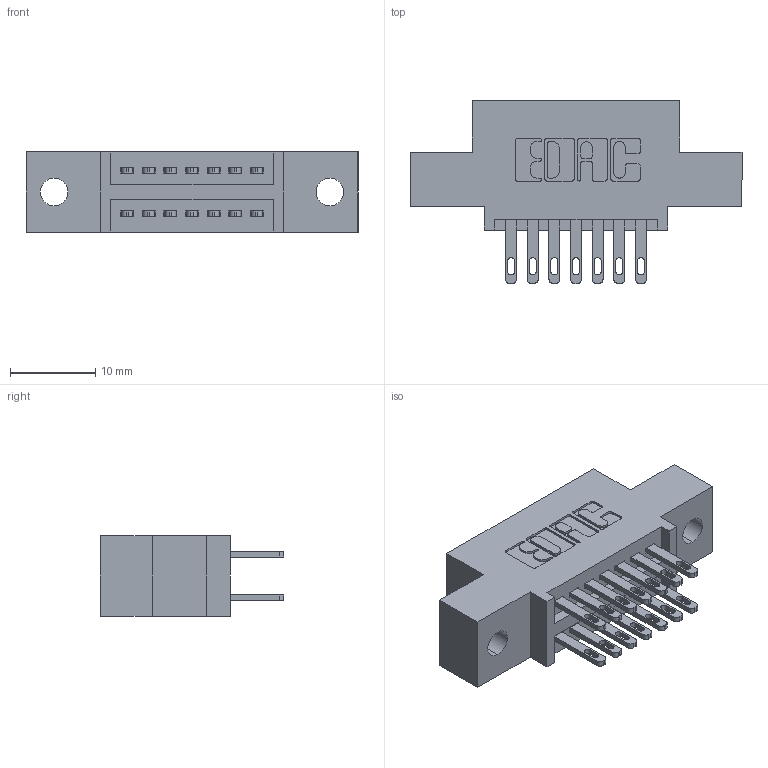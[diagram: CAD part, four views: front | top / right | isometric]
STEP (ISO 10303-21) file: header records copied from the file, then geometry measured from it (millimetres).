
FILE_DESCRIPTION (( 'STEP AP203' ), '1' );
FILE_NAME ('345-014-500-502.STEP', '2019-10-26T17:24:00', ( '' ), ( '' ), 'SwSTEP 2.0', 'SolidWorks 2016', '' );
FILE_SCHEMA (( 'CONFIG_CONTROL_DESIGN' ));
Length unit declared in the file: inch
Products named in the file (3): 345-292-001_345-293-100; 345-014-500-502; 345 Part_0.110 Offset - 0.128 Dia
Assembly tree (15 placements, depth 2):
  345-014-500-502
    345 Part_0.110 Offset - 0.128 Dia
    345-292-001_345-293-100  x14
Bounding box: 38.99 x 21.51 x 9.4 mm (x, y, z)
Volume: 3395.3 mm3; surface area: 4303.8 mm2
Topology: 15 solids, 15 shells, 774 faces, 2327 edges, 1550 vertices
Faces by surface type: plane 462, cylinder 312
Entity records: 10269 total; most frequent: CARTESIAN_POINT 1756, ORIENTED_EDGE 1690, DIRECTION 1593, EDGE_CURVE 845, LINE 681, VECTOR 681, VERTEX_POINT 562, AXIS2_PLACEMENT_3D 456
